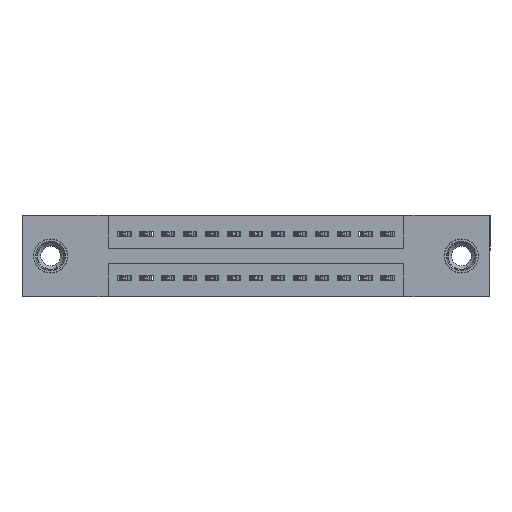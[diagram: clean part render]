
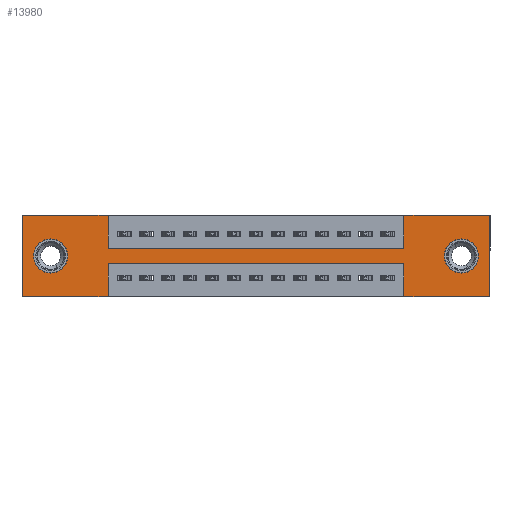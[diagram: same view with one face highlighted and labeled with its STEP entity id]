
A CAD part, front view. The second image highlights one B-rep face of the part: STEP entity #13980.
In plain terms, the highlighted planar face has unit normal (0, -1, 0).
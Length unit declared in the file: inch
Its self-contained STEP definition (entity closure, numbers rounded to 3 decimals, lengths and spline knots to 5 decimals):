
#7 = CARTESIAN_POINT ( 'NONE',  ( 0., 0., 0. ) ) ;
#34 = DIRECTION ( 'NONE',  ( 0., 0., 1. ) ) ;
#149 = CARTESIAN_POINT ( 'NONE',  ( 0.3925, 0., -0.22 ) ) ;
#164 = DIRECTION ( 'NONE',  ( 0., 0., 1. ) ) ;
#284 = EDGE_LOOP ( 'NONE', ( #16284, #13308 ) ) ;
#640 = DIRECTION ( 'NONE',  ( 0., 1., 0. ) ) ;
#674 = ORIENTED_EDGE ( 'NONE', *, *, #1725, .F. ) ;
#738 = ORIENTED_EDGE ( 'NONE', *, *, #5662, .F. ) ;
#837 = VERTEX_POINT ( 'NONE', #3862 ) ;
#998 = ORIENTED_EDGE ( 'NONE', *, *, #1341, .F. ) ;
#1008 = DIRECTION ( 'NONE',  ( 1., 0., 0. ) ) ;
#1337 = CARTESIAN_POINT ( 'NONE',  ( 0.13, 0., -0.185 ) ) ;
#1341 = EDGE_CURVE ( 'NONE', #837, #2191, #5407, .T. ) ;
#1366 = FACE_BOUND ( 'NONE', #4587, .T. ) ;
#1725 = EDGE_CURVE ( 'NONE', #2191, #6396, #3697, .T. ) ;
#2191 = VERTEX_POINT ( 'NONE', #4943 ) ;
#2208 = ORIENTED_EDGE ( 'NONE', *, *, #10927, .T. ) ;
#2260 = CIRCLE ( 'NONE', #11322, 0.078 ) ;
#2777 = CARTESIAN_POINT ( 'NONE',  ( 1.7425, 0., 0. ) ) ;
#2940 = DIRECTION ( 'NONE',  ( 0., 0., 1. ) ) ;
#3212 = DIRECTION ( 'NONE',  ( 0., 0., 1. ) ) ;
#3252 = CIRCLE ( 'NONE', #8330, 0.078 ) ;
#3371 = VERTEX_POINT ( 'NONE', #9858 ) ;
#3697 = LINE ( 'NONE', #2777, #14819 ) ;
#3862 = CARTESIAN_POINT ( 'NONE',  ( 0.3925, 0., -0.15 ) ) ;
#3945 = DIRECTION ( 'NONE',  ( 0., 0., -1. ) ) ;
#4292 = VERTEX_POINT ( 'NONE', #149 ) ;
#4372 = VERTEX_POINT ( 'NONE', #12449 ) ;
#4587 = EDGE_LOOP ( 'NONE', ( #2208, #4649 ) ) ;
#4649 = ORIENTED_EDGE ( 'NONE', *, *, #16817, .T. ) ;
#4690 = DIRECTION ( 'NONE',  ( 0., 0., 1. ) ) ;
#4882 = VECTOR ( 'NONE', #8164, 39.37008 ) ;
#4943 = CARTESIAN_POINT ( 'NONE',  ( 1.7425, 0., -0.15 ) ) ;
#4952 = DIRECTION ( 'NONE',  ( -1., 0., 0. ) ) ;
#5407 = LINE ( 'NONE', #6982, #12704 ) ;
#5457 = DIRECTION ( 'NONE',  ( 1., 0., 0. ) ) ;
#5535 = FACE_BOUND ( 'NONE', #284, .T. ) ;
#5662 = EDGE_CURVE ( 'NONE', #4292, #13866, #13435, .T. ) ;
#5833 = EDGE_CURVE ( 'NONE', #6870, #13056, #8274, .T. ) ;
#6186 = DIRECTION ( 'NONE',  ( 0., 0., -1. ) ) ;
#6218 = CARTESIAN_POINT ( 'NONE',  ( 0.13, 0., -0.263 ) ) ;
#6396 = VERTEX_POINT ( 'NONE', #17996 ) ;
#6689 = CARTESIAN_POINT ( 'NONE',  ( 0.3925, 0., -0.37 ) ) ;
#6739 = CARTESIAN_POINT ( 'NONE',  ( 2.005, 0., -0.185 ) ) ;
#6870 = VERTEX_POINT ( 'NONE', #9402 ) ;
#6905 = VECTOR ( 'NONE', #5457, 39.37008 ) ;
#6982 = CARTESIAN_POINT ( 'NONE',  ( 0.3925, 0., -0.15 ) ) ;
#7030 = VECTOR ( 'NONE', #4952, 39.37008 ) ;
#7500 = CARTESIAN_POINT ( 'NONE',  ( 2.135, 0., 0. ) ) ;
#7505 = AXIS2_PLACEMENT_3D ( 'NONE', #6739, #16664, #8192 ) ;
#7906 = AXIS2_PLACEMENT_3D ( 'NONE', #9760, #640, #11209 ) ;
#8032 = VECTOR ( 'NONE', #4690, 39.37008 ) ;
#8164 = DIRECTION ( 'NONE',  ( -1., 0., 0. ) ) ;
#8192 = DIRECTION ( 'NONE',  ( 0., 0., -1. ) ) ;
#8274 = LINE ( 'NONE', #8352, #6905 ) ;
#8280 = CARTESIAN_POINT ( 'NONE',  ( 2.005, 0., -0.263 ) ) ;
#8330 = AXIS2_PLACEMENT_3D ( 'NONE', #1337, #11810, #2940 ) ;
#8352 = CARTESIAN_POINT ( 'NONE',  ( 0., 0., 0. ) ) ;
#8436 = VECTOR ( 'NONE', #11423, 39.37008 ) ;
#8444 = EDGE_LOOP ( 'NONE', ( #738, #8633, #17870, #18707, #12257, #9795, #674, #998, #11060, #9621, #9915, #8879 ) ) ;
#8633 = ORIENTED_EDGE ( 'NONE', *, *, #11521, .F. ) ;
#8801 = VERTEX_POINT ( 'NONE', #17604 ) ;
#8841 = LINE ( 'NONE', #18034, #4882 ) ;
#8879 = ORIENTED_EDGE ( 'NONE', *, *, #18248, .F. ) ;
#8978 = FACE_OUTER_BOUND ( 'NONE', #8444, .T. ) ;
#9064 = EDGE_CURVE ( 'NONE', #13134, #6870, #16633, .T. ) ;
#9110 = CARTESIAN_POINT ( 'NONE',  ( 1.7425, 0., -0.37 ) ) ;
#9310 = DIRECTION ( 'NONE',  ( 0., 1., 0. ) ) ;
#9386 = CARTESIAN_POINT ( 'NONE',  ( 0., 0., -0.37 ) ) ;
#9402 = CARTESIAN_POINT ( 'NONE',  ( 0., 0., 0. ) ) ;
#9621 = ORIENTED_EDGE ( 'NONE', *, *, #5833, .F. ) ;
#9665 = AXIS2_PLACEMENT_3D ( 'NONE', #18246, #12775, #3945 ) ;
#9668 = VECTOR ( 'NONE', #12154, 39.37008 ) ;
#9760 = CARTESIAN_POINT ( 'NONE',  ( 2.005, 0., -0.185 ) ) ;
#9795 = ORIENTED_EDGE ( 'NONE', *, *, #16687, .F. ) ;
#9808 = EDGE_CURVE ( 'NONE', #18829, #4372, #12740, .T. ) ;
#9858 = CARTESIAN_POINT ( 'NONE',  ( 2.135, 0., -0.37 ) ) ;
#9915 = ORIENTED_EDGE ( 'NONE', *, *, #9064, .F. ) ;
#10017 = CARTESIAN_POINT ( 'NONE',  ( 1.7425, 0., -0.37 ) ) ;
#10080 = CARTESIAN_POINT ( 'NONE',  ( 0., 0., 0. ) ) ;
#10518 = EDGE_CURVE ( 'NONE', #3371, #11164, #16378, .T. ) ;
#10633 = CIRCLE ( 'NONE', #7906, 0.078 ) ;
#10704 = CARTESIAN_POINT ( 'NONE',  ( 0.3925, 0., -0.37 ) ) ;
#10927 = EDGE_CURVE ( 'NONE', #8801, #17602, #2260, .T. ) ;
#11060 = ORIENTED_EDGE ( 'NONE', *, *, #11415, .F. ) ;
#11164 = VERTEX_POINT ( 'NONE', #10017 ) ;
#11171 = CARTESIAN_POINT ( 'NONE',  ( 2.135, 0., 0. ) ) ;
#11209 = DIRECTION ( 'NONE',  ( 0., 0., -1. ) ) ;
#11277 = PLANE ( 'NONE',  #9665 ) ;
#11322 = AXIS2_PLACEMENT_3D ( 'NONE', #17705, #9310, #164 ) ;
#11415 = EDGE_CURVE ( 'NONE', #13056, #837, #15922, .T. ) ;
#11423 = DIRECTION ( 'NONE',  ( -1., 0., 0. ) ) ;
#11521 = EDGE_CURVE ( 'NONE', #11713, #4292, #18302, .T. ) ;
#11713 = VERTEX_POINT ( 'NONE', #16730 ) ;
#11810 = DIRECTION ( 'NONE',  ( 0., 1., 0. ) ) ;
#11956 = EDGE_CURVE ( 'NONE', #18261, #3371, #18283, .T. ) ;
#12034 = CARTESIAN_POINT ( 'NONE',  ( 0.3925, 0., 0. ) ) ;
#12154 = DIRECTION ( 'NONE',  ( 0., 0., -1. ) ) ;
#12237 = EDGE_CURVE ( 'NONE', #4372, #18829, #10633, .T. ) ;
#12251 = VECTOR ( 'NONE', #6186, 39.37008 ) ;
#12257 = ORIENTED_EDGE ( 'NONE', *, *, #11956, .F. ) ;
#12449 = CARTESIAN_POINT ( 'NONE',  ( 2.005, 0., -0.107 ) ) ;
#12704 = VECTOR ( 'NONE', #15138, 39.37008 ) ;
#12740 = CIRCLE ( 'NONE', #7505, 0.078 ) ;
#12775 = DIRECTION ( 'NONE',  ( 0., -1., 0. ) ) ;
#12973 = VECTOR ( 'NONE', #3212, 39.37008 ) ;
#13056 = VERTEX_POINT ( 'NONE', #12034 ) ;
#13134 = VERTEX_POINT ( 'NONE', #9386 ) ;
#13308 = ORIENTED_EDGE ( 'NONE', *, *, #9808, .T. ) ;
#13435 = LINE ( 'NONE', #10704, #9668 ) ;
#13866 = VERTEX_POINT ( 'NONE', #6689 ) ;
#13980 = ADVANCED_FACE ( 'NONE', ( #5535, #1366, #8978 ), #11277, .T. ) ;
#14612 = VECTOR ( 'NONE', #14687, 39.37008 ) ;
#14687 = DIRECTION ( 'NONE',  ( 0., 0., -1. ) ) ;
#14819 = VECTOR ( 'NONE', #34, 39.37008 ) ;
#15031 = CARTESIAN_POINT ( 'NONE',  ( 0.3925, 0., -0.22 ) ) ;
#15138 = DIRECTION ( 'NONE',  ( 1., 0., 0. ) ) ;
#15259 = EDGE_CURVE ( 'NONE', #11164, #11713, #16020, .T. ) ;
#15922 = LINE ( 'NONE', #17571, #12251 ) ;
#16020 = LINE ( 'NONE', #9110, #8032 ) ;
#16284 = ORIENTED_EDGE ( 'NONE', *, *, #12237, .T. ) ;
#16378 = LINE ( 'NONE', #18332, #8436 ) ;
#16610 = VECTOR ( 'NONE', #1008, 39.37008 ) ;
#16633 = LINE ( 'NONE', #7, #12973 ) ;
#16664 = DIRECTION ( 'NONE',  ( 0., 1., 0. ) ) ;
#16687 = EDGE_CURVE ( 'NONE', #6396, #18261, #17038, .T. ) ;
#16730 = CARTESIAN_POINT ( 'NONE',  ( 1.7425, 0., -0.22 ) ) ;
#16817 = EDGE_CURVE ( 'NONE', #17602, #8801, #3252, .T. ) ;
#17038 = LINE ( 'NONE', #10080, #16610 ) ;
#17571 = CARTESIAN_POINT ( 'NONE',  ( 0.3925, 0., 0. ) ) ;
#17602 = VERTEX_POINT ( 'NONE', #6218 ) ;
#17604 = CARTESIAN_POINT ( 'NONE',  ( 0.13, 0., -0.107 ) ) ;
#17705 = CARTESIAN_POINT ( 'NONE',  ( 0.13, 0., -0.185 ) ) ;
#17870 = ORIENTED_EDGE ( 'NONE', *, *, #15259, .F. ) ;
#17996 = CARTESIAN_POINT ( 'NONE',  ( 1.7425, 0., 0. ) ) ;
#18034 = CARTESIAN_POINT ( 'NONE',  ( 0., 0., -0.37 ) ) ;
#18246 = CARTESIAN_POINT ( 'NONE',  ( 0., 0., -0.37 ) ) ;
#18248 = EDGE_CURVE ( 'NONE', #13866, #13134, #8841, .T. ) ;
#18261 = VERTEX_POINT ( 'NONE', #11171 ) ;
#18283 = LINE ( 'NONE', #7500, #14612 ) ;
#18302 = LINE ( 'NONE', #15031, #7030 ) ;
#18332 = CARTESIAN_POINT ( 'NONE',  ( 0., 0., -0.37 ) ) ;
#18707 = ORIENTED_EDGE ( 'NONE', *, *, #10518, .F. ) ;
#18829 = VERTEX_POINT ( 'NONE', #8280 ) ;
